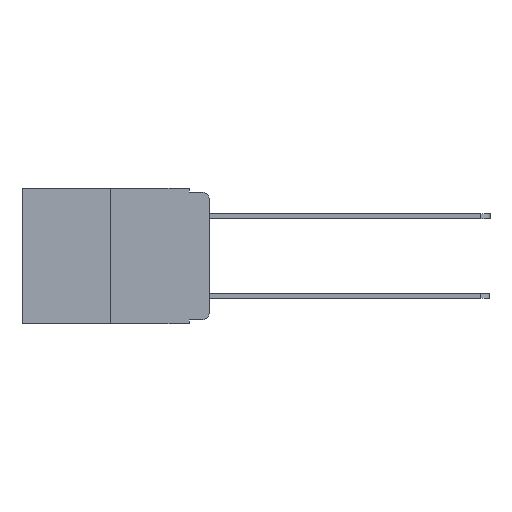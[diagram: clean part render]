
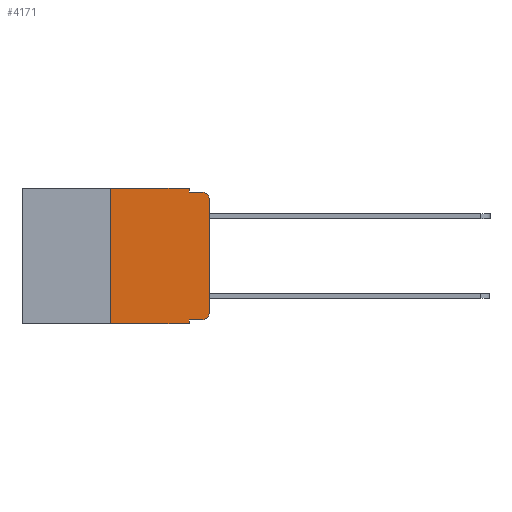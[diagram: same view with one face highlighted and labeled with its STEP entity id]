
A CAD part, left-side view. The second image highlights one B-rep face of the part: STEP entity #4171.
In plain terms, the highlighted planar face has unit normal (-1, 0, 0).
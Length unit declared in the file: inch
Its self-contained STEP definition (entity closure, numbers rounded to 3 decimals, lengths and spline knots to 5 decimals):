
#227 = EDGE_CURVE ( 'NONE', #2705, #11727, #3004, .T. ) ;
#414 = DIRECTION ( 'NONE',  ( 0., 0., -1. ) ) ;
#775 = ORIENTED_EDGE ( 'NONE', *, *, #14922, .T. ) ;
#935 = VERTEX_POINT ( 'NONE', #16567 ) ;
#996 = VERTEX_POINT ( 'NONE', #17565 ) ;
#1266 = VECTOR ( 'NONE', #3853, 39.37008 ) ;
#1533 = EDGE_CURVE ( 'NONE', #18230, #996, #9217, .T. ) ;
#1793 = DIRECTION ( 'NONE',  ( 0., 0., 1. ) ) ;
#1856 = LINE ( 'NONE', #14335, #16886 ) ;
#2029 = ORIENTED_EDGE ( 'NONE', *, *, #6333, .F. ) ;
#2303 = LINE ( 'NONE', #7382, #5931 ) ;
#2678 = CARTESIAN_POINT ( 'NONE',  ( 0., 0.02, -0.313 ) ) ;
#2705 = VERTEX_POINT ( 'NONE', #11737 ) ;
#2722 = EDGE_CURVE ( 'NONE', #17475, #935, #18094, .T. ) ;
#2805 = VERTEX_POINT ( 'NONE', #3688 ) ;
#3004 = LINE ( 'NONE', #4390, #17965 ) ;
#3323 = DIRECTION ( 'NONE',  ( 0., 0., -1. ) ) ;
#3332 = CARTESIAN_POINT ( 'NONE',  ( 0., 0.25, 0. ) ) ;
#3461 = ORIENTED_EDGE ( 'NONE', *, *, #1533, .F. ) ;
#3558 = DIRECTION ( 'NONE',  ( 1., 0., 0. ) ) ;
#3688 = CARTESIAN_POINT ( 'NONE',  ( 0., 0.25, 0. ) ) ;
#3853 = DIRECTION ( 'NONE',  ( 0., 0., 1. ) ) ;
#4171 = ADVANCED_FACE ( 'NONE', ( #5548 ), #12276, .F. ) ;
#4182 = ORIENTED_EDGE ( 'NONE', *, *, #12672, .F. ) ;
#4232 = DIRECTION ( 'NONE',  ( 0., 0., -1. ) ) ;
#4390 = CARTESIAN_POINT ( 'NONE',  ( 0., 0.051, 0. ) ) ;
#5072 = EDGE_CURVE ( 'NONE', #14984, #996, #1856, .T. ) ;
#5253 = DIRECTION ( 'NONE',  ( 0., -1., 0. ) ) ;
#5291 = EDGE_CURVE ( 'NONE', #18230, #7378, #8646, .T. ) ;
#5418 = AXIS2_PLACEMENT_3D ( 'NONE', #17960, #3558, #13730 ) ;
#5548 = FACE_OUTER_BOUND ( 'NONE', #18679, .T. ) ;
#5931 = VECTOR ( 'NONE', #17302, 39.37008 ) ;
#5944 = CARTESIAN_POINT ( 'NONE',  ( 0., 0.25, -0.343 ) ) ;
#6333 = EDGE_CURVE ( 'NONE', #14984, #2805, #11511, .T. ) ;
#6411 = DIRECTION ( 'NONE',  ( 0., -1., 0. ) ) ;
#6794 = CARTESIAN_POINT ( 'NONE',  ( 0., 0.02, -0.333 ) ) ;
#6804 = ORIENTED_EDGE ( 'NONE', *, *, #10048, .T. ) ;
#6927 = CARTESIAN_POINT ( 'NONE',  ( 0., 0., 0. ) ) ;
#7378 = VERTEX_POINT ( 'NONE', #6794 ) ;
#7382 = CARTESIAN_POINT ( 'NONE',  ( 0., 0.473, 0. ) ) ;
#7838 = LINE ( 'NONE', #13847, #14952 ) ;
#8646 = LINE ( 'NONE', #14940, #16197 ) ;
#8656 = DIRECTION ( 'NONE',  ( 0., -1., 0. ) ) ;
#8705 = CARTESIAN_POINT ( 'NONE',  ( 0., 0., -0.313 ) ) ;
#9016 = ORIENTED_EDGE ( 'NONE', *, *, #227, .F. ) ;
#9217 = LINE ( 'NONE', #10646, #17243 ) ;
#9415 = DIRECTION ( 'NONE',  ( -1., 0., 0. ) ) ;
#9452 = ORIENTED_EDGE ( 'NONE', *, *, #15645, .F. ) ;
#10048 = EDGE_CURVE ( 'NONE', #10250, #17475, #13043, .T. ) ;
#10250 = VERTEX_POINT ( 'NONE', #8705 ) ;
#10350 = ORIENTED_EDGE ( 'NONE', *, *, #5072, .T. ) ;
#10646 = CARTESIAN_POINT ( 'NONE',  ( 0., 0.051, 0. ) ) ;
#11004 = ORIENTED_EDGE ( 'NONE', *, *, #2722, .T. ) ;
#11063 = VECTOR ( 'NONE', #1793, 39.37008 ) ;
#11511 = LINE ( 'NONE', #3332, #11063 ) ;
#11727 = VERTEX_POINT ( 'NONE', #16404 ) ;
#11737 = CARTESIAN_POINT ( 'NONE',  ( 0., 0.051, 0. ) ) ;
#12276 = PLANE ( 'NONE',  #5418 ) ;
#12672 = EDGE_CURVE ( 'NONE', #11727, #935, #7838, .T. ) ;
#12923 = DIRECTION ( 'NONE',  ( -1., 0., 0. ) ) ;
#12993 = CARTESIAN_POINT ( 'NONE',  ( 0., 0.051, -0.333 ) ) ;
#13043 = LINE ( 'NONE', #6927, #1266 ) ;
#13432 = AXIS2_PLACEMENT_3D ( 'NONE', #17957, #9415, #414 ) ;
#13730 = DIRECTION ( 'NONE',  ( 0., 0., -1. ) ) ;
#13847 = CARTESIAN_POINT ( 'NONE',  ( 0., 0.051, -0.01 ) ) ;
#14094 = CARTESIAN_POINT ( 'NONE',  ( 0., 0., -0.03 ) ) ;
#14335 = CARTESIAN_POINT ( 'NONE',  ( 0., 0.473, -0.343 ) ) ;
#14663 = CIRCLE ( 'NONE', #17729, 0.02 ) ;
#14922 = EDGE_CURVE ( 'NONE', #7378, #10250, #14663, .T. ) ;
#14940 = CARTESIAN_POINT ( 'NONE',  ( 0., 0.051, -0.333 ) ) ;
#14952 = VECTOR ( 'NONE', #5253, 39.37008 ) ;
#14984 = VERTEX_POINT ( 'NONE', #5944 ) ;
#15478 = ORIENTED_EDGE ( 'NONE', *, *, #5291, .T. ) ;
#15645 = EDGE_CURVE ( 'NONE', #2805, #2705, #2303, .T. ) ;
#16197 = VECTOR ( 'NONE', #6411, 39.37008 ) ;
#16404 = CARTESIAN_POINT ( 'NONE',  ( 0., 0.051, -0.01 ) ) ;
#16504 = DIRECTION ( 'NONE',  ( 0., 0., -1. ) ) ;
#16567 = CARTESIAN_POINT ( 'NONE',  ( 0., 0.02, -0.01 ) ) ;
#16886 = VECTOR ( 'NONE', #8656, 39.37008 ) ;
#17243 = VECTOR ( 'NONE', #16504, 39.37008 ) ;
#17302 = DIRECTION ( 'NONE',  ( 0., -1., 0. ) ) ;
#17475 = VERTEX_POINT ( 'NONE', #14094 ) ;
#17565 = CARTESIAN_POINT ( 'NONE',  ( 0., 0.051, -0.343 ) ) ;
#17729 = AXIS2_PLACEMENT_3D ( 'NONE', #2678, #12923, #4232 ) ;
#17957 = CARTESIAN_POINT ( 'NONE',  ( 0., 0.02, -0.03 ) ) ;
#17960 = CARTESIAN_POINT ( 'NONE',  ( 0., 0.473, 0. ) ) ;
#17965 = VECTOR ( 'NONE', #3323, 39.37008 ) ;
#18094 = CIRCLE ( 'NONE', #13432, 0.02 ) ;
#18230 = VERTEX_POINT ( 'NONE', #12993 ) ;
#18679 = EDGE_LOOP ( 'NONE', ( #6804, #11004, #4182, #9016, #9452, #2029, #10350, #3461, #15478, #775 ) ) ;
